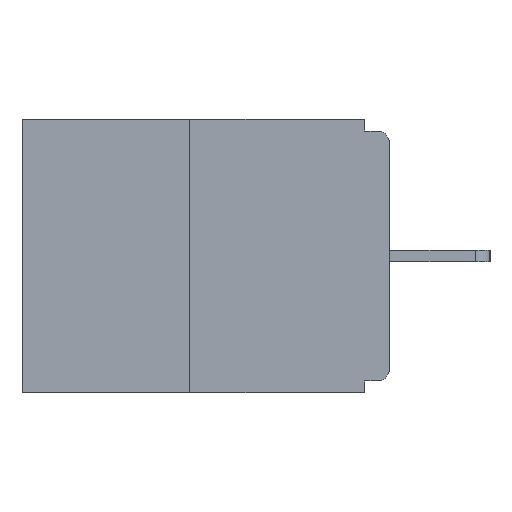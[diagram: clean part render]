
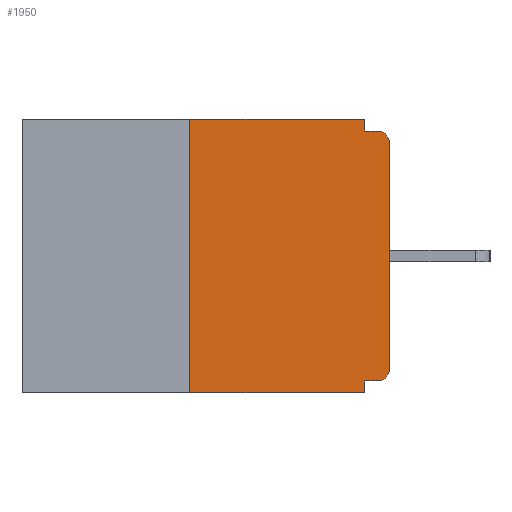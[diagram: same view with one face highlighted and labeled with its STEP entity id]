
A CAD part, left-side view. The second image highlights one B-rep face of the part: STEP entity #1950.
In plain terms, the highlighted planar face has unit normal (-1, 0, 0).
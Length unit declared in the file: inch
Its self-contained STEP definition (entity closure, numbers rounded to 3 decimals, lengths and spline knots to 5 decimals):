
#62 = EDGE_CURVE ( 'NONE', #3648, #1530, #21478, .T. ) ;
#522 = CARTESIAN_POINT ( 'NONE',  ( 0., 0.031, -0.343 ) ) ;
#859 = EDGE_CURVE ( 'NONE', #21474, #25094, #25854, .T. ) ;
#1206 = EDGE_CURVE ( 'NONE', #8584, #3648, #15094, .T. ) ;
#1530 = VERTEX_POINT ( 'NONE', #8275 ) ;
#1782 = ORIENTED_EDGE ( 'NONE', *, *, #14012, .F. ) ;
#1848 = ORIENTED_EDGE ( 'NONE', *, *, #1206, .T. ) ;
#1950 = ADVANCED_FACE ( 'NONE', ( #21871 ), #18058, .F. ) ;
#2031 = DIRECTION ( 'NONE',  ( 0., -1., 0. ) ) ;
#2555 = CARTESIAN_POINT ( 'NONE',  ( 0., 0.015, -0.015 ) ) ;
#2837 = CARTESIAN_POINT ( 'NONE',  ( 0., 0.031, -0.328 ) ) ;
#2947 = CARTESIAN_POINT ( 'NONE',  ( 0., 0.25, 0. ) ) ;
#3053 = LINE ( 'NONE', #23349, #8442 ) ;
#3317 = DIRECTION ( 'NONE',  ( 0., 1., 0. ) ) ;
#3366 = ORIENTED_EDGE ( 'NONE', *, *, #5170, .F. ) ;
#3648 = VERTEX_POINT ( 'NONE', #23972 ) ;
#4248 = CARTESIAN_POINT ( 'NONE',  ( 0., 0.015, -0.328 ) ) ;
#5065 = CARTESIAN_POINT ( 'NONE',  ( 0., 0.031, -0.015 ) ) ;
#5170 = EDGE_CURVE ( 'NONE', #8584, #13078, #3053, .T. ) ;
#5264 = DIRECTION ( 'NONE',  ( 0., 0., -1. ) ) ;
#5781 = EDGE_CURVE ( 'NONE', #13078, #20543, #21760, .T. ) ;
#5886 = CARTESIAN_POINT ( 'NONE',  ( 0., 0., 0. ) ) ;
#6094 = CARTESIAN_POINT ( 'NONE',  ( 0., 0.031, 0. ) ) ;
#7289 = ORIENTED_EDGE ( 'NONE', *, *, #15562, .T. ) ;
#7524 = DIRECTION ( 'NONE',  ( 0., 0., 1. ) ) ;
#8098 = CARTESIAN_POINT ( 'NONE',  ( 0., 0.25, -0.343 ) ) ;
#8196 = CARTESIAN_POINT ( 'NONE',  ( 0., 0.46, 0. ) ) ;
#8252 = CARTESIAN_POINT ( 'NONE',  ( 0., 0.46, 0. ) ) ;
#8275 = CARTESIAN_POINT ( 'NONE',  ( 0., 0., -0.03 ) ) ;
#8435 = LINE ( 'NONE', #8196, #22846 ) ;
#8442 = VECTOR ( 'NONE', #3317, 39.37008 ) ;
#8562 = CIRCLE ( 'NONE', #20701, 0.015 ) ;
#8584 = VERTEX_POINT ( 'NONE', #4248 ) ;
#8683 = LINE ( 'NONE', #24922, #19634 ) ;
#10412 = ORIENTED_EDGE ( 'NONE', *, *, #5781, .F. ) ;
#10978 = VECTOR ( 'NONE', #11771, 39.37008 ) ;
#11447 = CARTESIAN_POINT ( 'NONE',  ( 0., 0.25, 0. ) ) ;
#11454 = VERTEX_POINT ( 'NONE', #6094 ) ;
#11749 = CARTESIAN_POINT ( 'NONE',  ( 0., 0.46, -0.343 ) ) ;
#11771 = DIRECTION ( 'NONE',  ( 0., 0., 1. ) ) ;
#12658 = ORIENTED_EDGE ( 'NONE', *, *, #13906, .F. ) ;
#12728 = AXIS2_PLACEMENT_3D ( 'NONE', #8252, #16214, #24202 ) ;
#12736 = CARTESIAN_POINT ( 'NONE',  ( 0., 0.015, -0.313 ) ) ;
#13019 = VECTOR ( 'NONE', #25677, 39.37008 ) ;
#13078 = VERTEX_POINT ( 'NONE', #2837 ) ;
#13085 = VERTEX_POINT ( 'NONE', #5065 ) ;
#13906 = EDGE_CURVE ( 'NONE', #11454, #13085, #18885, .T. ) ;
#14012 = EDGE_CURVE ( 'NONE', #13085, #16330, #8683, .T. ) ;
#14809 = DIRECTION ( 'NONE',  ( -1., 0., 0. ) ) ;
#14812 = CARTESIAN_POINT ( 'NONE',  ( 0., 0.031, 0. ) ) ;
#15094 = CIRCLE ( 'NONE', #15525, 0.015 ) ;
#15525 = AXIS2_PLACEMENT_3D ( 'NONE', #12736, #14809, #5264 ) ;
#15562 = EDGE_CURVE ( 'NONE', #1530, #16330, #8562, .T. ) ;
#16127 = CARTESIAN_POINT ( 'NONE',  ( 0., 0.015, -0.03 ) ) ;
#16214 = DIRECTION ( 'NONE',  ( 1., 0., 0. ) ) ;
#16330 = VERTEX_POINT ( 'NONE', #2555 ) ;
#17804 = CARTESIAN_POINT ( 'NONE',  ( 0., 0.031, -0.343 ) ) ;
#17901 = LINE ( 'NONE', #11749, #20375 ) ;
#17918 = ORIENTED_EDGE ( 'NONE', *, *, #21983, .F. ) ;
#18058 = PLANE ( 'NONE',  #12728 ) ;
#18885 = LINE ( 'NONE', #14812, #20938 ) ;
#19016 = DIRECTION ( 'NONE',  ( 0., 0., -1. ) ) ;
#19244 = ORIENTED_EDGE ( 'NONE', *, *, #859, .F. ) ;
#19598 = EDGE_CURVE ( 'NONE', #21474, #20543, #17901, .T. ) ;
#19634 = VECTOR ( 'NONE', #22566, 39.37008 ) ;
#20151 = EDGE_LOOP ( 'NONE', ( #17918, #19244, #21836, #10412, #3366, #1848, #24276, #7289, #1782, #12658 ) ) ;
#20375 = VECTOR ( 'NONE', #24177, 39.37008 ) ;
#20543 = VERTEX_POINT ( 'NONE', #522 ) ;
#20701 = AXIS2_PLACEMENT_3D ( 'NONE', #16127, #24119, #22152 ) ;
#20938 = VECTOR ( 'NONE', #19016, 39.37008 ) ;
#21474 = VERTEX_POINT ( 'NONE', #8098 ) ;
#21478 = LINE ( 'NONE', #5886, #10978 ) ;
#21760 = LINE ( 'NONE', #17804, #13019 ) ;
#21836 = ORIENTED_EDGE ( 'NONE', *, *, #19598, .T. ) ;
#21871 = FACE_OUTER_BOUND ( 'NONE', #20151, .T. ) ;
#21983 = EDGE_CURVE ( 'NONE', #25094, #11454, #8435, .T. ) ;
#22152 = DIRECTION ( 'NONE',  ( 0., 0., -1. ) ) ;
#22566 = DIRECTION ( 'NONE',  ( 0., -1., 0. ) ) ;
#22846 = VECTOR ( 'NONE', #2031, 39.37008 ) ;
#23349 = CARTESIAN_POINT ( 'NONE',  ( 0., 0., -0.328 ) ) ;
#23972 = CARTESIAN_POINT ( 'NONE',  ( 0., 0., -0.313 ) ) ;
#24119 = DIRECTION ( 'NONE',  ( -1., 0., 0. ) ) ;
#24177 = DIRECTION ( 'NONE',  ( 0., -1., 0. ) ) ;
#24202 = DIRECTION ( 'NONE',  ( 0., 0., -1. ) ) ;
#24276 = ORIENTED_EDGE ( 'NONE', *, *, #62, .T. ) ;
#24922 = CARTESIAN_POINT ( 'NONE',  ( 0., 0., -0.015 ) ) ;
#25094 = VERTEX_POINT ( 'NONE', #2947 ) ;
#25096 = VECTOR ( 'NONE', #7524, 39.37008 ) ;
#25677 = DIRECTION ( 'NONE',  ( 0., 0., -1. ) ) ;
#25854 = LINE ( 'NONE', #11447, #25096 ) ;
